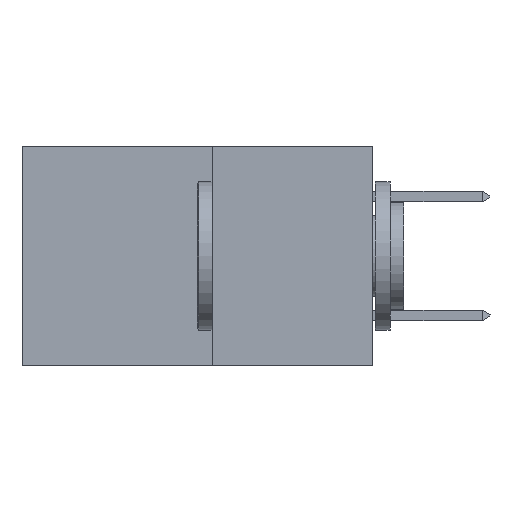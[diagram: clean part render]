
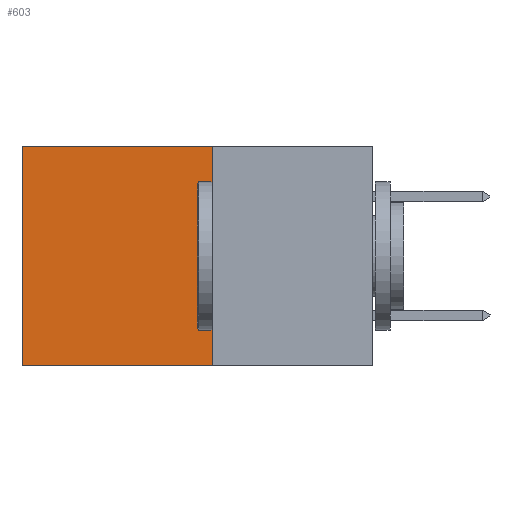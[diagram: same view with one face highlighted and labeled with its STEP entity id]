
A CAD part, left-side view. The second image highlights one B-rep face of the part: STEP entity #603.
In plain terms, the highlighted planar face has unit normal (-1, 0, 0).
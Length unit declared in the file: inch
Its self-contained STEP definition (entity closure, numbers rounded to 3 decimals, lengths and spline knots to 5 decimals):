
#55 = VECTOR ( 'NONE', #24063, 39.37008 ) ;
#603 = ADVANCED_FACE ( 'NONE', ( #17661 ), #8749, .F. ) ;
#1448 = VERTEX_POINT ( 'NONE', #21299 ) ;
#2080 = CARTESIAN_POINT ( 'NONE',  ( 0.277, 0.27, -0.37 ) ) ;
#2467 = VECTOR ( 'NONE', #23643, 39.37008 ) ;
#3308 = CARTESIAN_POINT ( 'NONE',  ( 0.277, 0.27, -0.37 ) ) ;
#4558 = EDGE_CURVE ( 'NONE', #1448, #14432, #24300, .T. ) ;
#4899 = CARTESIAN_POINT ( 'NONE',  ( 0.277, 0.27, -0.37 ) ) ;
#5100 = CARTESIAN_POINT ( 'NONE',  ( 0.277, 0.59, 0. ) ) ;
#5731 = VERTEX_POINT ( 'NONE', #11041 ) ;
#5744 = ORIENTED_EDGE ( 'NONE', *, *, #24507, .T. ) ;
#6221 = EDGE_CURVE ( 'NONE', #14432, #5731, #17650, .T. ) ;
#6366 = ORIENTED_EDGE ( 'NONE', *, *, #4558, .F. ) ;
#8522 = DIRECTION ( 'NONE',  ( 0., 0., -1. ) ) ;
#8655 = DIRECTION ( 'NONE',  ( 1., 0., 0. ) ) ;
#8681 = EDGE_CURVE ( 'NONE', #1448, #21745, #21134, .T. ) ;
#8749 = PLANE ( 'NONE',  #14039 ) ;
#9240 = DIRECTION ( 'NONE',  ( 0., 0., -1. ) ) ;
#11041 = CARTESIAN_POINT ( 'NONE',  ( 0.277, 0.59, -0.37 ) ) ;
#12928 = ORIENTED_EDGE ( 'NONE', *, *, #6221, .F. ) ;
#14039 = AXIS2_PLACEMENT_3D ( 'NONE', #4899, #8655, #8522 ) ;
#14432 = VERTEX_POINT ( 'NONE', #23848 ) ;
#16577 = VECTOR ( 'NONE', #9240, 39.37008 ) ;
#17300 = LINE ( 'NONE', #20793, #16577 ) ;
#17650 = LINE ( 'NONE', #3308, #23808 ) ;
#17661 = FACE_OUTER_BOUND ( 'NONE', #26238, .T. ) ;
#19699 = DIRECTION ( 'NONE',  ( 0., 1., 0. ) ) ;
#20793 = CARTESIAN_POINT ( 'NONE',  ( 0.277, 0.59, -0.37 ) ) ;
#21134 = LINE ( 'NONE', #26001, #2467 ) ;
#21299 = CARTESIAN_POINT ( 'NONE',  ( 0.277, 0.27, 0. ) ) ;
#21745 = VERTEX_POINT ( 'NONE', #5100 ) ;
#23643 = DIRECTION ( 'NONE',  ( 0., 1., 0. ) ) ;
#23808 = VECTOR ( 'NONE', #19699, 39.37008 ) ;
#23848 = CARTESIAN_POINT ( 'NONE',  ( 0.277, 0.27, -0.37 ) ) ;
#24063 = DIRECTION ( 'NONE',  ( 0., 0., -1. ) ) ;
#24300 = LINE ( 'NONE', #2080, #55 ) ;
#24507 = EDGE_CURVE ( 'NONE', #21745, #5731, #17300, .T. ) ;
#26001 = CARTESIAN_POINT ( 'NONE',  ( 0.277, 0.27, 0. ) ) ;
#26238 = EDGE_LOOP ( 'NONE', ( #5744, #12928, #6366, #26698 ) ) ;
#26698 = ORIENTED_EDGE ( 'NONE', *, *, #8681, .T. ) ;
